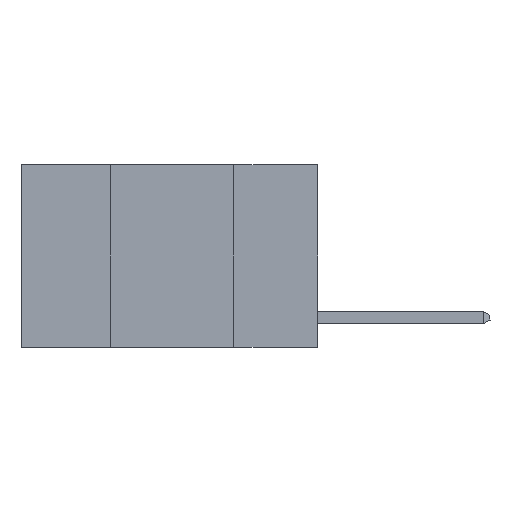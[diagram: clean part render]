
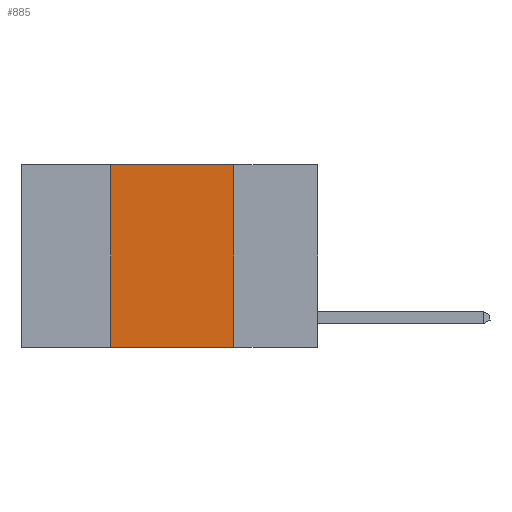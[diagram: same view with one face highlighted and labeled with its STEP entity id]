
A CAD part, left-side view. The second image highlights one B-rep face of the part: STEP entity #885.
In plain terms, the highlighted planar face has unit normal (-1, 0, 0).
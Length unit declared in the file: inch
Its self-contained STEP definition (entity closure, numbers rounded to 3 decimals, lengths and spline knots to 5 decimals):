
#885 = ADVANCED_FACE ( 'NONE', ( #5991 ), #5226, .F. ) ;
#1066 = CARTESIAN_POINT ( 'NONE',  ( 0., 0.6, 0. ) ) ;
#1368 = EDGE_CURVE ( 'NONE', #1667, #21696, #9498, .T. ) ;
#1514 = VECTOR ( 'NONE', #7201, 39.37008 ) ;
#1667 = VERTEX_POINT ( 'NONE', #15782 ) ;
#1719 = VECTOR ( 'NONE', #2735, 39.37008 ) ;
#2017 = VERTEX_POINT ( 'NONE', #16656 ) ;
#2735 = DIRECTION ( 'NONE',  ( 0., 0., -1. ) ) ;
#2828 = DIRECTION ( 'NONE',  ( 0., -1., 0. ) ) ;
#4423 = EDGE_CURVE ( 'NONE', #1667, #2017, #15872, .T. ) ;
#4880 = VECTOR ( 'NONE', #16686, 39.37008 ) ;
#5226 = PLANE ( 'NONE',  #14981 ) ;
#5456 = CARTESIAN_POINT ( 'NONE',  ( 0., 0.6, -0.37 ) ) ;
#5763 = EDGE_LOOP ( 'NONE', ( #19785, #18511, #17286, #18625 ) ) ;
#5991 = FACE_OUTER_BOUND ( 'NONE', #5763, .T. ) ;
#6316 = LINE ( 'NONE', #9650, #1719 ) ;
#6328 = CARTESIAN_POINT ( 'NONE',  ( 0., 0.42, 0. ) ) ;
#6368 = CARTESIAN_POINT ( 'NONE',  ( 0., 0.42, 0. ) ) ;
#6872 = LINE ( 'NONE', #1066, #19594 ) ;
#6978 = DIRECTION ( 'NONE',  ( 1., 0., 0. ) ) ;
#7138 = VERTEX_POINT ( 'NONE', #7983 ) ;
#7201 = DIRECTION ( 'NONE',  ( 0., -1., 0. ) ) ;
#7983 = CARTESIAN_POINT ( 'NONE',  ( 0., 0.17, 0. ) ) ;
#9498 = LINE ( 'NONE', #6328, #4880 ) ;
#9505 = EDGE_CURVE ( 'NONE', #7138, #2017, #6316, .T. ) ;
#9650 = CARTESIAN_POINT ( 'NONE',  ( 0., 0.17, 0. ) ) ;
#11794 = EDGE_CURVE ( 'NONE', #21696, #7138, #6872, .T. ) ;
#12122 = CARTESIAN_POINT ( 'NONE',  ( 0., 0.6, 0. ) ) ;
#14981 = AXIS2_PLACEMENT_3D ( 'NONE', #12122, #6978, #19102 ) ;
#15782 = CARTESIAN_POINT ( 'NONE',  ( 0., 0.42, -0.37 ) ) ;
#15872 = LINE ( 'NONE', #5456, #1514 ) ;
#16656 = CARTESIAN_POINT ( 'NONE',  ( 0., 0.17, -0.37 ) ) ;
#16686 = DIRECTION ( 'NONE',  ( 0., 0., 1. ) ) ;
#17286 = ORIENTED_EDGE ( 'NONE', *, *, #1368, .F. ) ;
#18511 = ORIENTED_EDGE ( 'NONE', *, *, #11794, .F. ) ;
#18625 = ORIENTED_EDGE ( 'NONE', *, *, #4423, .T. ) ;
#19102 = DIRECTION ( 'NONE',  ( 0., 0., -1. ) ) ;
#19594 = VECTOR ( 'NONE', #2828, 39.37008 ) ;
#19785 = ORIENTED_EDGE ( 'NONE', *, *, #9505, .F. ) ;
#21696 = VERTEX_POINT ( 'NONE', #6368 ) ;
